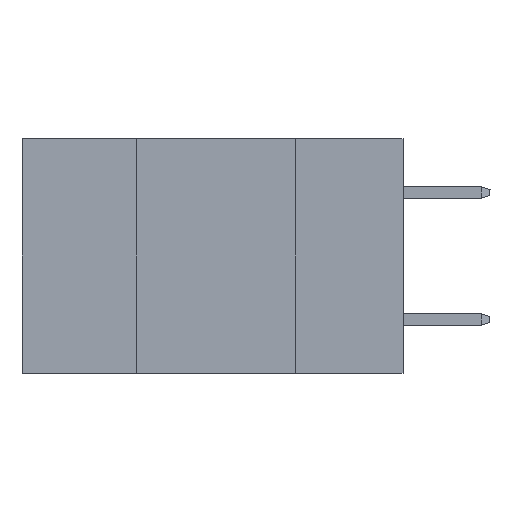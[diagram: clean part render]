
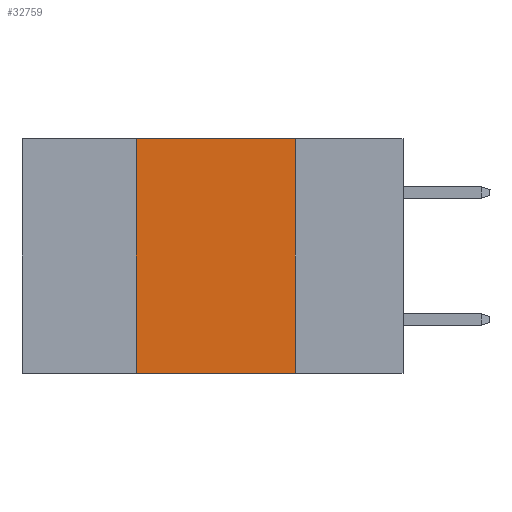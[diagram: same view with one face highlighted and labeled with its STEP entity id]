
A CAD part, left-side view. The second image highlights one B-rep face of the part: STEP entity #32759.
In plain terms, the highlighted planar face has unit normal (-1, 0, 0).
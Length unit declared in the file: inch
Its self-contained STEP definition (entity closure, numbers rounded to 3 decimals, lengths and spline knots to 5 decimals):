
#175 = CARTESIAN_POINT ( 'NONE',  ( 0., 0.17, 0. ) ) ;
#1004 = VERTEX_POINT ( 'NONE', #40861 ) ;
#1106 = ORIENTED_EDGE ( 'NONE', *, *, #14182, .F. ) ;
#2207 = CARTESIAN_POINT ( 'NONE',  ( 0., 0.6, 0. ) ) ;
#2587 = CARTESIAN_POINT ( 'NONE',  ( 0., 0.42, 0. ) ) ;
#4071 = EDGE_LOOP ( 'NONE', ( #35911, #38052, #1106, #39057 ) ) ;
#4301 = EDGE_CURVE ( 'NONE', #24581, #29329, #29110, .T. ) ;
#5035 = DIRECTION ( 'NONE',  ( 0., 0., -1. ) ) ;
#5561 = CARTESIAN_POINT ( 'NONE',  ( 0., 0.42, -0.37 ) ) ;
#6346 = LINE ( 'NONE', #13467, #20271 ) ;
#11336 = DIRECTION ( 'NONE',  ( 1., 0., 0. ) ) ;
#13467 = CARTESIAN_POINT ( 'NONE',  ( 0., 0.6, -0.37 ) ) ;
#13609 = DIRECTION ( 'NONE',  ( 0., 0., -1. ) ) ;
#14059 = VECTOR ( 'NONE', #36402, 39.37008 ) ;
#14182 = EDGE_CURVE ( 'NONE', #21440, #24581, #23388, .T. ) ;
#14985 = EDGE_CURVE ( 'NONE', #21440, #1004, #6346, .T. ) ;
#16157 = VECTOR ( 'NONE', #13609, 39.37008 ) ;
#18562 = AXIS2_PLACEMENT_3D ( 'NONE', #34098, #11336, #5035 ) ;
#18779 = VECTOR ( 'NONE', #19376, 39.37008 ) ;
#19376 = DIRECTION ( 'NONE',  ( 0., -1., 0. ) ) ;
#19896 = CARTESIAN_POINT ( 'NONE',  ( 0., 0.42, 0. ) ) ;
#20271 = VECTOR ( 'NONE', #22827, 39.37008 ) ;
#21440 = VERTEX_POINT ( 'NONE', #5561 ) ;
#22827 = DIRECTION ( 'NONE',  ( 0., -1., 0. ) ) ;
#23388 = LINE ( 'NONE', #2587, #14059 ) ;
#23453 = CARTESIAN_POINT ( 'NONE',  ( 0., 0.17, 0. ) ) ;
#24581 = VERTEX_POINT ( 'NONE', #19896 ) ;
#29110 = LINE ( 'NONE', #2207, #18779 ) ;
#29329 = VERTEX_POINT ( 'NONE', #23453 ) ;
#32725 = LINE ( 'NONE', #175, #16157 ) ;
#32759 = ADVANCED_FACE ( 'NONE', ( #34308 ), #34733, .F. ) ;
#34098 = CARTESIAN_POINT ( 'NONE',  ( 0., 0.6, 0. ) ) ;
#34308 = FACE_OUTER_BOUND ( 'NONE', #4071, .T. ) ;
#34733 = PLANE ( 'NONE',  #18562 ) ;
#35911 = ORIENTED_EDGE ( 'NONE', *, *, #36692, .F. ) ;
#36402 = DIRECTION ( 'NONE',  ( 0., 0., 1. ) ) ;
#36692 = EDGE_CURVE ( 'NONE', #29329, #1004, #32725, .T. ) ;
#38052 = ORIENTED_EDGE ( 'NONE', *, *, #4301, .F. ) ;
#39057 = ORIENTED_EDGE ( 'NONE', *, *, #14985, .T. ) ;
#40861 = CARTESIAN_POINT ( 'NONE',  ( 0., 0.17, -0.37 ) ) ;
